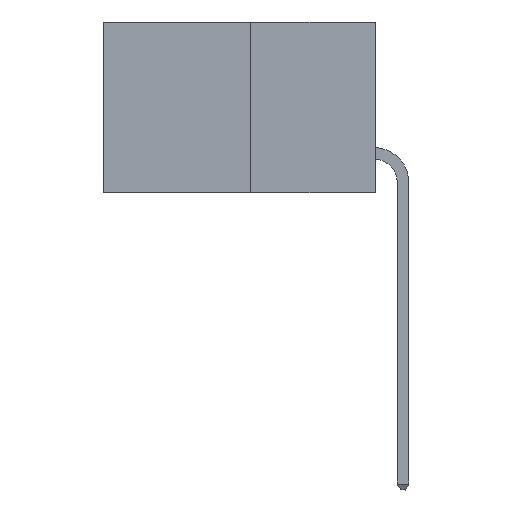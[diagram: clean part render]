
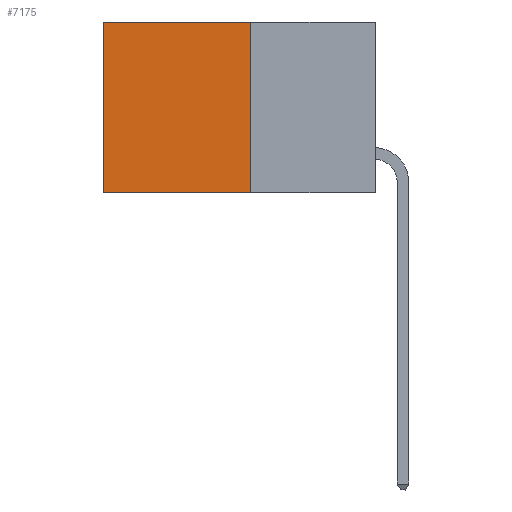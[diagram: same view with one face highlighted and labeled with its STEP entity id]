
A CAD part, left-side view. The second image highlights one B-rep face of the part: STEP entity #7175.
In plain terms, the highlighted planar face has unit normal (-1, 0, 0).
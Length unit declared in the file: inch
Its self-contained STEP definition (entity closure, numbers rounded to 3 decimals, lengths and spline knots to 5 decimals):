
#693 = EDGE_CURVE ( 'NONE', #16450, #15450, #3343, .T. ) ;
#1075 = ORIENTED_EDGE ( 'NONE', *, *, #12699, .F. ) ;
#2582 = VERTEX_POINT ( 'NONE', #14359 ) ;
#3205 = DIRECTION ( 'NONE',  ( 0., 0., -1. ) ) ;
#3343 = LINE ( 'NONE', #10506, #6961 ) ;
#3521 = EDGE_LOOP ( 'NONE', ( #18309, #1075, #7688, #7792 ) ) ;
#4526 = AXIS2_PLACEMENT_3D ( 'NONE', #10754, #6279, #3205 ) ;
#5032 = FACE_OUTER_BOUND ( 'NONE', #3521, .T. ) ;
#6044 = CARTESIAN_POINT ( 'NONE',  ( 0.277, 0.59, -0.37 ) ) ;
#6238 = VECTOR ( 'NONE', #18224, 39.37008 ) ;
#6279 = DIRECTION ( 'NONE',  ( 1., 0., 0. ) ) ;
#6961 = VECTOR ( 'NONE', #10438, 39.37008 ) ;
#7175 = ADVANCED_FACE ( 'NONE', ( #5032 ), #12249, .F. ) ;
#7494 = VECTOR ( 'NONE', #14898, 39.37008 ) ;
#7688 = ORIENTED_EDGE ( 'NONE', *, *, #11333, .F. ) ;
#7792 = ORIENTED_EDGE ( 'NONE', *, *, #693, .T. ) ;
#7961 = CARTESIAN_POINT ( 'NONE',  ( 0.277, 0.27, -0.37 ) ) ;
#8140 = LINE ( 'NONE', #17467, #15560 ) ;
#8374 = CARTESIAN_POINT ( 'NONE',  ( 0.277, 0.27, 0. ) ) ;
#9084 = VERTEX_POINT ( 'NONE', #7961 ) ;
#10076 = DIRECTION ( 'NONE',  ( 0., 0., -1. ) ) ;
#10298 = EDGE_CURVE ( 'NONE', #15450, #2582, #11454, .T. ) ;
#10438 = DIRECTION ( 'NONE',  ( 0., 1., 0. ) ) ;
#10506 = CARTESIAN_POINT ( 'NONE',  ( 0.277, 0.27, 0. ) ) ;
#10754 = CARTESIAN_POINT ( 'NONE',  ( 0.277, 0.27, -0.37 ) ) ;
#11333 = EDGE_CURVE ( 'NONE', #16450, #9084, #8140, .T. ) ;
#11454 = LINE ( 'NONE', #6044, #7494 ) ;
#12249 = PLANE ( 'NONE',  #4526 ) ;
#12699 = EDGE_CURVE ( 'NONE', #9084, #2582, #14120, .T. ) ;
#14120 = LINE ( 'NONE', #16772, #6238 ) ;
#14359 = CARTESIAN_POINT ( 'NONE',  ( 0.277, 0.59, -0.37 ) ) ;
#14898 = DIRECTION ( 'NONE',  ( 0., 0., -1. ) ) ;
#15025 = CARTESIAN_POINT ( 'NONE',  ( 0.277, 0.59, 0. ) ) ;
#15450 = VERTEX_POINT ( 'NONE', #15025 ) ;
#15560 = VECTOR ( 'NONE', #10076, 39.37008 ) ;
#16450 = VERTEX_POINT ( 'NONE', #8374 ) ;
#16772 = CARTESIAN_POINT ( 'NONE',  ( 0.277, 0.27, -0.37 ) ) ;
#17467 = CARTESIAN_POINT ( 'NONE',  ( 0.277, 0.27, -0.37 ) ) ;
#18224 = DIRECTION ( 'NONE',  ( 0., 1., 0. ) ) ;
#18309 = ORIENTED_EDGE ( 'NONE', *, *, #10298, .T. ) ;
